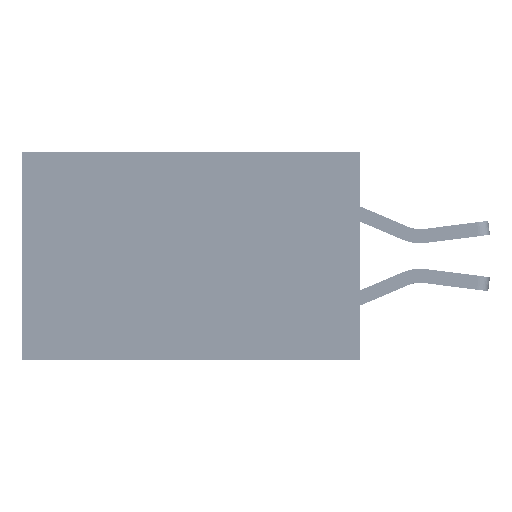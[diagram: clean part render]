
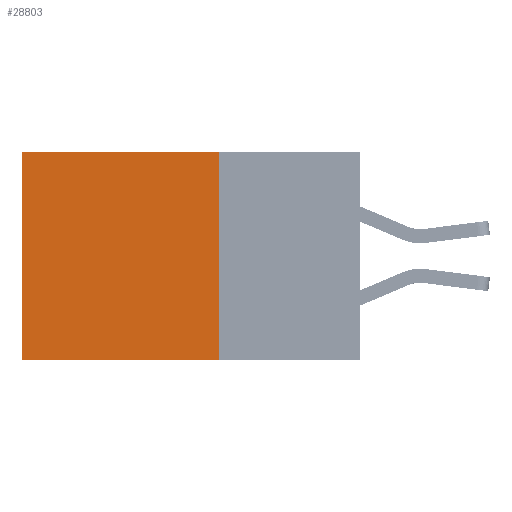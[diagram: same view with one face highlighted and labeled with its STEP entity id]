
A CAD part, left-side view. The second image highlights one B-rep face of the part: STEP entity #28803.
In plain terms, the highlighted planar face has unit normal (-1, 0, 0).
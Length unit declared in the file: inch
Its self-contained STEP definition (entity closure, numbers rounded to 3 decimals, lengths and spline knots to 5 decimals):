
#272 = VERTEX_POINT ( 'NONE', #20665 ) ;
#521 = EDGE_CURVE ( 'NONE', #272, #24409, #11588, .T. ) ;
#1185 = CARTESIAN_POINT ( 'NONE',  ( 0.2875, 0.25, -0.37 ) ) ;
#1363 = DIRECTION ( 'NONE',  ( 0., 0., -1. ) ) ;
#1739 = VECTOR ( 'NONE', #28598, 39.37008 ) ;
#2355 = CARTESIAN_POINT ( 'NONE',  ( 0.2875, 0.6, 0. ) ) ;
#3690 = LINE ( 'NONE', #2355, #5769 ) ;
#4764 = CARTESIAN_POINT ( 'NONE',  ( 0.2875, 0.25, 0. ) ) ;
#5769 = VECTOR ( 'NONE', #41879, 39.37008 ) ;
#7888 = DIRECTION ( 'NONE',  ( 1., 0., 0. ) ) ;
#7984 = LINE ( 'NONE', #35122, #1739 ) ;
#8901 = ORIENTED_EDGE ( 'NONE', *, *, #9188, .F. ) ;
#9175 = CARTESIAN_POINT ( 'NONE',  ( 0.2875, 0.6, 0. ) ) ;
#9188 = EDGE_CURVE ( 'NONE', #36738, #27898, #7984, .T. ) ;
#10425 = CARTESIAN_POINT ( 'NONE',  ( 0.2875, 0.6, -0.37 ) ) ;
#10940 = CARTESIAN_POINT ( 'NONE',  ( 0.2875, 0.25, 0. ) ) ;
#11433 = DIRECTION ( 'NONE',  ( 0., 1., 0. ) ) ;
#11588 = LINE ( 'NONE', #4764, #38703 ) ;
#14236 = FACE_OUTER_BOUND ( 'NONE', #17726, .T. ) ;
#16246 = EDGE_CURVE ( 'NONE', #24409, #27898, #3690, .T. ) ;
#17726 = EDGE_LOOP ( 'NONE', ( #35669, #8901, #33683, #24236 ) ) ;
#20665 = CARTESIAN_POINT ( 'NONE',  ( 0.2875, 0.25, 0. ) ) ;
#21443 = AXIS2_PLACEMENT_3D ( 'NONE', #40922, #7888, #1363 ) ;
#24236 = ORIENTED_EDGE ( 'NONE', *, *, #521, .T. ) ;
#24409 = VERTEX_POINT ( 'NONE', #9175 ) ;
#27171 = VECTOR ( 'NONE', #40172, 39.37008 ) ;
#27898 = VERTEX_POINT ( 'NONE', #10425 ) ;
#28598 = DIRECTION ( 'NONE',  ( 0., 1., 0. ) ) ;
#28803 = ADVANCED_FACE ( 'NONE', ( #14236 ), #31489, .F. ) ;
#31489 = PLANE ( 'NONE',  #21443 ) ;
#33683 = ORIENTED_EDGE ( 'NONE', *, *, #37754, .F. ) ;
#35122 = CARTESIAN_POINT ( 'NONE',  ( 0.2875, 0.25, -0.37 ) ) ;
#35669 = ORIENTED_EDGE ( 'NONE', *, *, #16246, .T. ) ;
#36023 = LINE ( 'NONE', #10940, #27171 ) ;
#36738 = VERTEX_POINT ( 'NONE', #1185 ) ;
#37754 = EDGE_CURVE ( 'NONE', #272, #36738, #36023, .T. ) ;
#38703 = VECTOR ( 'NONE', #11433, 39.37008 ) ;
#40172 = DIRECTION ( 'NONE',  ( 0., 0., -1. ) ) ;
#40922 = CARTESIAN_POINT ( 'NONE',  ( 0.2875, 0.25, 0. ) ) ;
#41879 = DIRECTION ( 'NONE',  ( 0., 0., -1. ) ) ;
